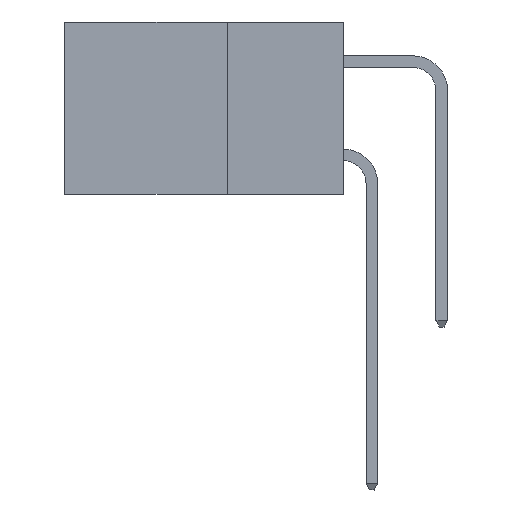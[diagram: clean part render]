
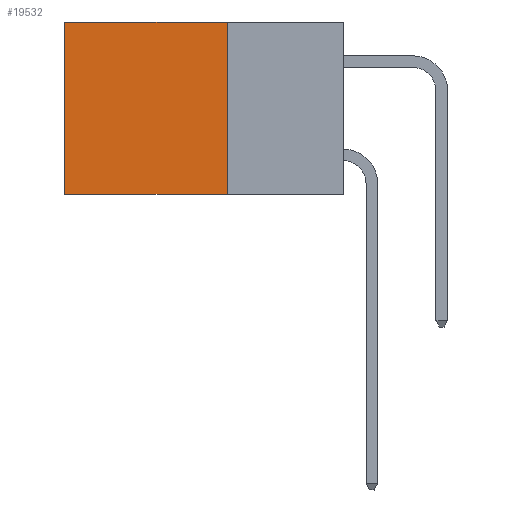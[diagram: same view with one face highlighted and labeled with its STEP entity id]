
A CAD part, left-side view. The second image highlights one B-rep face of the part: STEP entity #19532.
In plain terms, the highlighted planar face has unit normal (-1, 0, 0).
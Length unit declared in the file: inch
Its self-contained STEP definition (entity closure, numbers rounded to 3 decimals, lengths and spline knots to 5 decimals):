
#263 = FACE_OUTER_BOUND ( 'NONE', #25131, .T. ) ;
#539 = ORIENTED_EDGE ( 'NONE', *, *, #12814, .F. ) ;
#717 = VECTOR ( 'NONE', #26630, 39.37008 ) ;
#795 = EDGE_CURVE ( 'NONE', #27103, #7358, #2283, .T. ) ;
#990 = DIRECTION ( 'NONE',  ( 0., 1., 0. ) ) ;
#1221 = CARTESIAN_POINT ( 'NONE',  ( 0.298, 0.25, 0. ) ) ;
#1896 = ORIENTED_EDGE ( 'NONE', *, *, #23349, .T. ) ;
#2283 = LINE ( 'NONE', #11675, #13524 ) ;
#2864 = LINE ( 'NONE', #3056, #21740 ) ;
#3056 = CARTESIAN_POINT ( 'NONE',  ( 0.298, 0.25, 0. ) ) ;
#3370 = DIRECTION ( 'NONE',  ( 1., 0., 0. ) ) ;
#3412 = EDGE_CURVE ( 'NONE', #15303, #26775, #18578, .T. ) ;
#3703 = DIRECTION ( 'NONE',  ( 0., 0., -1. ) ) ;
#7127 = DIRECTION ( 'NONE',  ( 0., 1., 0. ) ) ;
#7358 = VERTEX_POINT ( 'NONE', #13252 ) ;
#9919 = ORIENTED_EDGE ( 'NONE', *, *, #3412, .F. ) ;
#10398 = DIRECTION ( 'NONE',  ( 0., 0., -1. ) ) ;
#11675 = CARTESIAN_POINT ( 'NONE',  ( 0.298, 0.6, 0. ) ) ;
#12814 = EDGE_CURVE ( 'NONE', #26775, #7358, #21610, .T. ) ;
#13252 = CARTESIAN_POINT ( 'NONE',  ( 0.298, 0.6, -0.37 ) ) ;
#13524 = VECTOR ( 'NONE', #3703, 39.37008 ) ;
#15303 = VERTEX_POINT ( 'NONE', #22455 ) ;
#15659 = VECTOR ( 'NONE', #7127, 39.37008 ) ;
#16943 = CARTESIAN_POINT ( 'NONE',  ( 0.298, 0.6, 0. ) ) ;
#18578 = LINE ( 'NONE', #22085, #717 ) ;
#19532 = ADVANCED_FACE ( 'NONE', ( #263 ), #28098, .F. ) ;
#20502 = CARTESIAN_POINT ( 'NONE',  ( 0.298, 0.25, -0.37 ) ) ;
#21610 = LINE ( 'NONE', #20502, #15659 ) ;
#21740 = VECTOR ( 'NONE', #990, 39.37008 ) ;
#21851 = ORIENTED_EDGE ( 'NONE', *, *, #795, .T. ) ;
#22085 = CARTESIAN_POINT ( 'NONE',  ( 0.298, 0.25, 0. ) ) ;
#22373 = CARTESIAN_POINT ( 'NONE',  ( 0.298, 0.25, -0.37 ) ) ;
#22455 = CARTESIAN_POINT ( 'NONE',  ( 0.298, 0.25, 0. ) ) ;
#23349 = EDGE_CURVE ( 'NONE', #15303, #27103, #2864, .T. ) ;
#24064 = AXIS2_PLACEMENT_3D ( 'NONE', #1221, #3370, #10398 ) ;
#25131 = EDGE_LOOP ( 'NONE', ( #21851, #539, #9919, #1896 ) ) ;
#26630 = DIRECTION ( 'NONE',  ( 0., 0., -1. ) ) ;
#26775 = VERTEX_POINT ( 'NONE', #22373 ) ;
#27103 = VERTEX_POINT ( 'NONE', #16943 ) ;
#28098 = PLANE ( 'NONE',  #24064 ) ;
